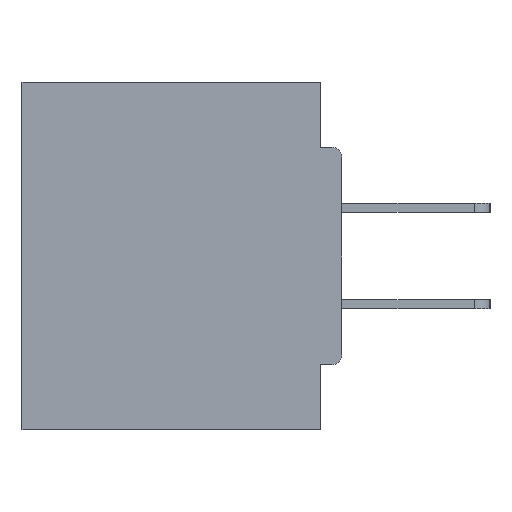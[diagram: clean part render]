
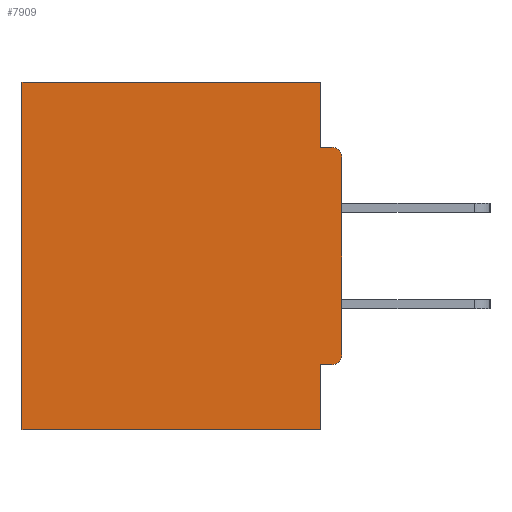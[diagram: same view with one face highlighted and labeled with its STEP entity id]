
A CAD part, left-side view. The second image highlights one B-rep face of the part: STEP entity #7909.
In plain terms, the highlighted planar face has unit normal (-1, 0, 0).
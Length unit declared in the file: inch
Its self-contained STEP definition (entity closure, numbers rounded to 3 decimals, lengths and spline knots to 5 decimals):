
#138 = DIRECTION ( 'NONE',  ( 0., 1., 0. ) ) ;
#2139 = EDGE_CURVE ( 'NONE', #35945, #35097, #32976, .T. ) ;
#2587 = LINE ( 'NONE', #18010, #20002 ) ;
#2623 = CARTESIAN_POINT ( 'NONE',  ( 0.298, 0.031, -0.5 ) ) ;
#3056 = VECTOR ( 'NONE', #37564, 39.37008 ) ;
#4469 = CARTESIAN_POINT ( 'NONE',  ( 0.298, 0.031, -0.4065 ) ) ;
#4846 = VECTOR ( 'NONE', #26705, 39.37008 ) ;
#4987 = PLANE ( 'NONE',  #44104 ) ;
#5137 = DIRECTION ( 'NONE',  ( 1., 0., 0. ) ) ;
#5693 = DIRECTION ( 'NONE',  ( 0., -1., 0. ) ) ;
#6562 = LINE ( 'NONE', #30050, #12553 ) ;
#6669 = VERTEX_POINT ( 'NONE', #38688 ) ;
#6862 = FACE_OUTER_BOUND ( 'NONE', #32464, .T. ) ;
#7241 = VERTEX_POINT ( 'NONE', #27554 ) ;
#7909 = ADVANCED_FACE ( 'NONE', ( #6862 ), #4987, .F. ) ;
#8078 = EDGE_CURVE ( 'NONE', #35945, #32261, #43341, .T. ) ;
#8869 = CARTESIAN_POINT ( 'NONE',  ( 0.298, 0.46, 0. ) ) ;
#9827 = ORIENTED_EDGE ( 'NONE', *, *, #11553, .F. ) ;
#10728 = DIRECTION ( 'NONE',  ( 0., 0., -1. ) ) ;
#11553 = EDGE_CURVE ( 'NONE', #29871, #14914, #6562, .T. ) ;
#12241 = VECTOR ( 'NONE', #43353, 39.37008 ) ;
#12553 = VECTOR ( 'NONE', #5693, 39.37008 ) ;
#13323 = VECTOR ( 'NONE', #33653, 39.37008 ) ;
#13431 = DIRECTION ( 'NONE',  ( -1., 0., 0. ) ) ;
#13941 = ORIENTED_EDGE ( 'NONE', *, *, #8078, .T. ) ;
#14652 = EDGE_CURVE ( 'NONE', #6669, #32261, #15496, .T. ) ;
#14726 = VECTOR ( 'NONE', #45028, 39.37008 ) ;
#14914 = VERTEX_POINT ( 'NONE', #30977 ) ;
#15496 = LINE ( 'NONE', #18976, #12241 ) ;
#15818 = CARTESIAN_POINT ( 'NONE',  ( 0.298, 0.015, -0.3915 ) ) ;
#16536 = CARTESIAN_POINT ( 'NONE',  ( 0.298, 0.031, -0.0935 ) ) ;
#17147 = CARTESIAN_POINT ( 'NONE',  ( 0.298, 0., -0.5 ) ) ;
#17400 = LINE ( 'NONE', #17147, #14726 ) ;
#17771 = LINE ( 'NONE', #8869, #3056 ) ;
#17829 = EDGE_CURVE ( 'NONE', #39435, #7241, #17400, .T. ) ;
#17904 = CARTESIAN_POINT ( 'NONE',  ( 0.298, 0., 0. ) ) ;
#18010 = CARTESIAN_POINT ( 'NONE',  ( 0.298, 0.031, -0.5 ) ) ;
#18976 = CARTESIAN_POINT ( 'NONE',  ( 0.298, 0., 0. ) ) ;
#19774 = AXIS2_PLACEMENT_3D ( 'NONE', #37484, #13431, #41253 ) ;
#20002 = VECTOR ( 'NONE', #10728, 39.37008 ) ;
#20698 = CARTESIAN_POINT ( 'NONE',  ( 0.298, 0.031, 0. ) ) ;
#21144 = VERTEX_POINT ( 'NONE', #20698 ) ;
#21987 = ORIENTED_EDGE ( 'NONE', *, *, #43863, .T. ) ;
#22623 = CARTESIAN_POINT ( 'NONE',  ( 0.298, 0., 0. ) ) ;
#23046 = ORIENTED_EDGE ( 'NONE', *, *, #35305, .T. ) ;
#23346 = CARTESIAN_POINT ( 'NONE',  ( 0.298, 0.031, -0.5 ) ) ;
#26328 = ORIENTED_EDGE ( 'NONE', *, *, #2139, .F. ) ;
#26335 = DIRECTION ( 'NONE',  ( 0., 0., -1. ) ) ;
#26705 = DIRECTION ( 'NONE',  ( 0., 0., -1. ) ) ;
#27234 = VECTOR ( 'NONE', #138, 39.37008 ) ;
#27554 = CARTESIAN_POINT ( 'NONE',  ( 0.298, 0.46, -0.5 ) ) ;
#27971 = EDGE_CURVE ( 'NONE', #35097, #39435, #2587, .T. ) ;
#28429 = ORIENTED_EDGE ( 'NONE', *, *, #41703, .T. ) ;
#29082 = ORIENTED_EDGE ( 'NONE', *, *, #14652, .F. ) ;
#29446 = LINE ( 'NONE', #17904, #27234 ) ;
#29871 = VERTEX_POINT ( 'NONE', #16536 ) ;
#30050 = CARTESIAN_POINT ( 'NONE',  ( 0.298, 0., -0.0935 ) ) ;
#30448 = CARTESIAN_POINT ( 'NONE',  ( 0.298, 0., -0.4065 ) ) ;
#30977 = CARTESIAN_POINT ( 'NONE',  ( 0.298, 0.015, -0.0935 ) ) ;
#32261 = VERTEX_POINT ( 'NONE', #40703 ) ;
#32464 = EDGE_LOOP ( 'NONE', ( #23046, #9827, #35069, #28429, #21987, #43939, #36715, #26328, #13941, #29082 ) ) ;
#32976 = LINE ( 'NONE', #30448, #13323 ) ;
#33116 = CARTESIAN_POINT ( 'NONE',  ( 0.298, 0.46, 0. ) ) ;
#33556 = EDGE_CURVE ( 'NONE', #21144, #29871, #41862, .T. ) ;
#33653 = DIRECTION ( 'NONE',  ( 0., 1., 0. ) ) ;
#35069 = ORIENTED_EDGE ( 'NONE', *, *, #33556, .F. ) ;
#35097 = VERTEX_POINT ( 'NONE', #4469 ) ;
#35305 = EDGE_CURVE ( 'NONE', #6669, #14914, #44443, .T. ) ;
#35945 = VERTEX_POINT ( 'NONE', #36858 ) ;
#36658 = DIRECTION ( 'NONE',  ( 0., 0., -1. ) ) ;
#36715 = ORIENTED_EDGE ( 'NONE', *, *, #27971, .F. ) ;
#36858 = CARTESIAN_POINT ( 'NONE',  ( 0.298, 0.015, -0.4065 ) ) ;
#37484 = CARTESIAN_POINT ( 'NONE',  ( 0.298, 0.015, -0.1085 ) ) ;
#37564 = DIRECTION ( 'NONE',  ( 0., 0., -1. ) ) ;
#37697 = AXIS2_PLACEMENT_3D ( 'NONE', #15818, #43700, #26335 ) ;
#38688 = CARTESIAN_POINT ( 'NONE',  ( 0.298, 0., -0.1085 ) ) ;
#39435 = VERTEX_POINT ( 'NONE', #2623 ) ;
#40459 = VERTEX_POINT ( 'NONE', #33116 ) ;
#40703 = CARTESIAN_POINT ( 'NONE',  ( 0.298, 0., -0.3915 ) ) ;
#41253 = DIRECTION ( 'NONE',  ( 0., 0., -1. ) ) ;
#41703 = EDGE_CURVE ( 'NONE', #21144, #40459, #29446, .T. ) ;
#41862 = LINE ( 'NONE', #23346, #4846 ) ;
#43341 = CIRCLE ( 'NONE', #37697, 0.015 ) ;
#43353 = DIRECTION ( 'NONE',  ( 0., 0., -1. ) ) ;
#43700 = DIRECTION ( 'NONE',  ( -1., 0., 0. ) ) ;
#43863 = EDGE_CURVE ( 'NONE', #40459, #7241, #17771, .T. ) ;
#43939 = ORIENTED_EDGE ( 'NONE', *, *, #17829, .F. ) ;
#44104 = AXIS2_PLACEMENT_3D ( 'NONE', #22623, #5137, #36658 ) ;
#44443 = CIRCLE ( 'NONE', #19774, 0.015 ) ;
#45028 = DIRECTION ( 'NONE',  ( 0., 1., 0. ) ) ;
